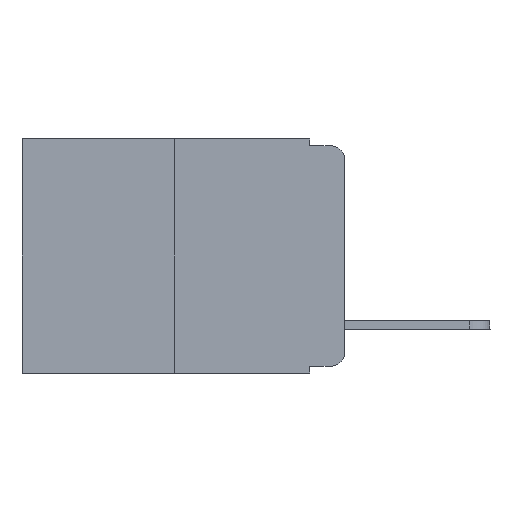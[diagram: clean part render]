
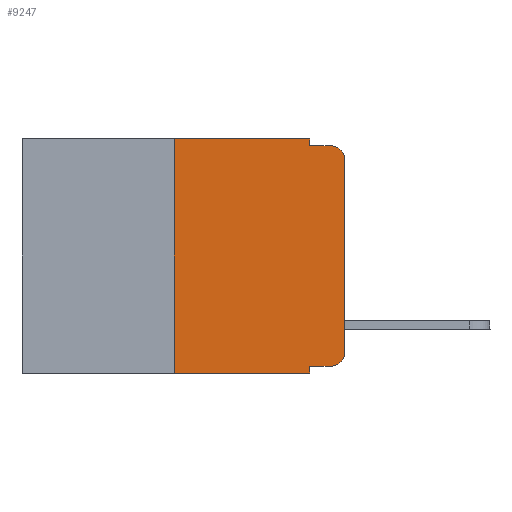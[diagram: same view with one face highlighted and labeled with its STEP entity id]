
A CAD part, left-side view. The second image highlights one B-rep face of the part: STEP entity #9247.
In plain terms, the highlighted planar face has unit normal (-1, 0, 0).
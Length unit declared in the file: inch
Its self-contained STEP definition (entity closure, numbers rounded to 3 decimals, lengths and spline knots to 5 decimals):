
#13 = VERTEX_POINT ( 'NONE', #9772 ) ;
#29 = ORIENTED_EDGE ( 'NONE', *, *, #5412, .F. ) ;
#220 = CARTESIAN_POINT ( 'NONE',  ( 0., 0.25, 0. ) ) ;
#268 = CARTESIAN_POINT ( 'NONE',  ( 0., 0.25, -0.343 ) ) ;
#371 = VERTEX_POINT ( 'NONE', #220 ) ;
#381 = DIRECTION ( 'NONE',  ( 1., 0., 0. ) ) ;
#572 = VERTEX_POINT ( 'NONE', #11095 ) ;
#587 = ORIENTED_EDGE ( 'NONE', *, *, #6769, .F. ) ;
#630 = EDGE_CURVE ( 'NONE', #2598, #3562, #11413, .T. ) ;
#692 = DIRECTION ( 'NONE',  ( 0., 0., -1. ) ) ;
#800 = CARTESIAN_POINT ( 'NONE',  ( 0., 0.02, -0.01 ) ) ;
#1224 = LINE ( 'NONE', #10804, #6529 ) ;
#1323 = CARTESIAN_POINT ( 'NONE',  ( 0., 0.02, -0.333 ) ) ;
#1332 = VECTOR ( 'NONE', #11593, 39.37008 ) ;
#1361 = CARTESIAN_POINT ( 'NONE',  ( 0., 0., 0. ) ) ;
#1656 = EDGE_CURVE ( 'NONE', #6640, #13, #5951, .T. ) ;
#1719 = DIRECTION ( 'NONE',  ( 0., 0., 1. ) ) ;
#1750 = ORIENTED_EDGE ( 'NONE', *, *, #4248, .T. ) ;
#1953 = EDGE_CURVE ( 'NONE', #3562, #3681, #9497, .T. ) ;
#2011 = VERTEX_POINT ( 'NONE', #8860 ) ;
#2055 = VECTOR ( 'NONE', #6914, 39.37008 ) ;
#2218 = VECTOR ( 'NONE', #2883, 39.37008 ) ;
#2230 = AXIS2_PLACEMENT_3D ( 'NONE', #10049, #381, #12026 ) ;
#2549 = DIRECTION ( 'NONE',  ( -1., 0., 0. ) ) ;
#2598 = VERTEX_POINT ( 'NONE', #6366 ) ;
#2883 = DIRECTION ( 'NONE',  ( 0., 0., 1. ) ) ;
#3236 = CARTESIAN_POINT ( 'NONE',  ( 0., 0.051, -0.01 ) ) ;
#3560 = CARTESIAN_POINT ( 'NONE',  ( 0., 0.02, -0.313 ) ) ;
#3562 = VERTEX_POINT ( 'NONE', #3236 ) ;
#3579 = CARTESIAN_POINT ( 'NONE',  ( 0., 0.051, 0. ) ) ;
#3681 = VERTEX_POINT ( 'NONE', #800 ) ;
#3719 = DIRECTION ( 'NONE',  ( 0., 0., -1. ) ) ;
#3722 = LINE ( 'NONE', #3907, #2218 ) ;
#3907 = CARTESIAN_POINT ( 'NONE',  ( 0., 0.25, 0. ) ) ;
#3917 = LINE ( 'NONE', #7103, #10354 ) ;
#4197 = VECTOR ( 'NONE', #12421, 39.37008 ) ;
#4248 = EDGE_CURVE ( 'NONE', #2011, #6561, #1224, .T. ) ;
#4698 = ORIENTED_EDGE ( 'NONE', *, *, #630, .F. ) ;
#5177 = PLANE ( 'NONE',  #2230 ) ;
#5247 = VECTOR ( 'NONE', #1719, 39.37008 ) ;
#5314 = AXIS2_PLACEMENT_3D ( 'NONE', #8080, #11007, #12201 ) ;
#5412 = EDGE_CURVE ( 'NONE', #2011, #13, #9568, .T. ) ;
#5610 = ORIENTED_EDGE ( 'NONE', *, *, #1953, .F. ) ;
#5951 = LINE ( 'NONE', #8001, #2055 ) ;
#6366 = CARTESIAN_POINT ( 'NONE',  ( 0., 0.051, 0. ) ) ;
#6529 = VECTOR ( 'NONE', #11637, 39.37008 ) ;
#6561 = VERTEX_POINT ( 'NONE', #1323 ) ;
#6640 = VERTEX_POINT ( 'NONE', #268 ) ;
#6658 = CIRCLE ( 'NONE', #8480, 0.02 ) ;
#6769 = EDGE_CURVE ( 'NONE', #371, #2598, #3917, .T. ) ;
#6886 = ORIENTED_EDGE ( 'NONE', *, *, #1656, .T. ) ;
#6914 = DIRECTION ( 'NONE',  ( 0., -1., 0. ) ) ;
#7103 = CARTESIAN_POINT ( 'NONE',  ( 0., 0.473, 0. ) ) ;
#7140 = FACE_OUTER_BOUND ( 'NONE', #9071, .T. ) ;
#7413 = EDGE_CURVE ( 'NONE', #12584, #572, #9403, .T. ) ;
#8001 = CARTESIAN_POINT ( 'NONE',  ( 0., 0.473, -0.343 ) ) ;
#8080 = CARTESIAN_POINT ( 'NONE',  ( 0., 0.02, -0.03 ) ) ;
#8480 = AXIS2_PLACEMENT_3D ( 'NONE', #3560, #2549, #692 ) ;
#8552 = CARTESIAN_POINT ( 'NONE',  ( 0., 0.051, -0.01 ) ) ;
#8860 = CARTESIAN_POINT ( 'NONE',  ( 0., 0.051, -0.333 ) ) ;
#8957 = VECTOR ( 'NONE', #3719, 39.37008 ) ;
#9071 = EDGE_LOOP ( 'NONE', ( #10467, #11867, #5610, #4698, #587, #11308, #6886, #29, #1750, #9650 ) ) ;
#9184 = CIRCLE ( 'NONE', #5314, 0.02 ) ;
#9247 = ADVANCED_FACE ( 'NONE', ( #7140 ), #5177, .F. ) ;
#9396 = EDGE_CURVE ( 'NONE', #6561, #12584, #6658, .T. ) ;
#9403 = LINE ( 'NONE', #1361, #5247 ) ;
#9497 = LINE ( 'NONE', #8552, #4197 ) ;
#9568 = LINE ( 'NONE', #12240, #8957 ) ;
#9650 = ORIENTED_EDGE ( 'NONE', *, *, #9396, .T. ) ;
#9772 = CARTESIAN_POINT ( 'NONE',  ( 0., 0.051, -0.343 ) ) ;
#9773 = EDGE_CURVE ( 'NONE', #6640, #371, #3722, .T. ) ;
#9881 = DIRECTION ( 'NONE',  ( 0., -1., 0. ) ) ;
#10049 = CARTESIAN_POINT ( 'NONE',  ( 0., 0.473, 0. ) ) ;
#10354 = VECTOR ( 'NONE', #9881, 39.37008 ) ;
#10467 = ORIENTED_EDGE ( 'NONE', *, *, #7413, .T. ) ;
#10804 = CARTESIAN_POINT ( 'NONE',  ( 0., 0.051, -0.333 ) ) ;
#11007 = DIRECTION ( 'NONE',  ( -1., 0., 0. ) ) ;
#11095 = CARTESIAN_POINT ( 'NONE',  ( 0., 0., -0.03 ) ) ;
#11308 = ORIENTED_EDGE ( 'NONE', *, *, #9773, .F. ) ;
#11413 = LINE ( 'NONE', #3579, #1332 ) ;
#11593 = DIRECTION ( 'NONE',  ( 0., 0., -1. ) ) ;
#11637 = DIRECTION ( 'NONE',  ( 0., -1., 0. ) ) ;
#11866 = CARTESIAN_POINT ( 'NONE',  ( 0., 0., -0.313 ) ) ;
#11867 = ORIENTED_EDGE ( 'NONE', *, *, #12234, .T. ) ;
#12026 = DIRECTION ( 'NONE',  ( 0., 0., -1. ) ) ;
#12201 = DIRECTION ( 'NONE',  ( 0., 0., -1. ) ) ;
#12234 = EDGE_CURVE ( 'NONE', #572, #3681, #9184, .T. ) ;
#12240 = CARTESIAN_POINT ( 'NONE',  ( 0., 0.051, 0. ) ) ;
#12421 = DIRECTION ( 'NONE',  ( 0., -1., 0. ) ) ;
#12584 = VERTEX_POINT ( 'NONE', #11866 ) ;
